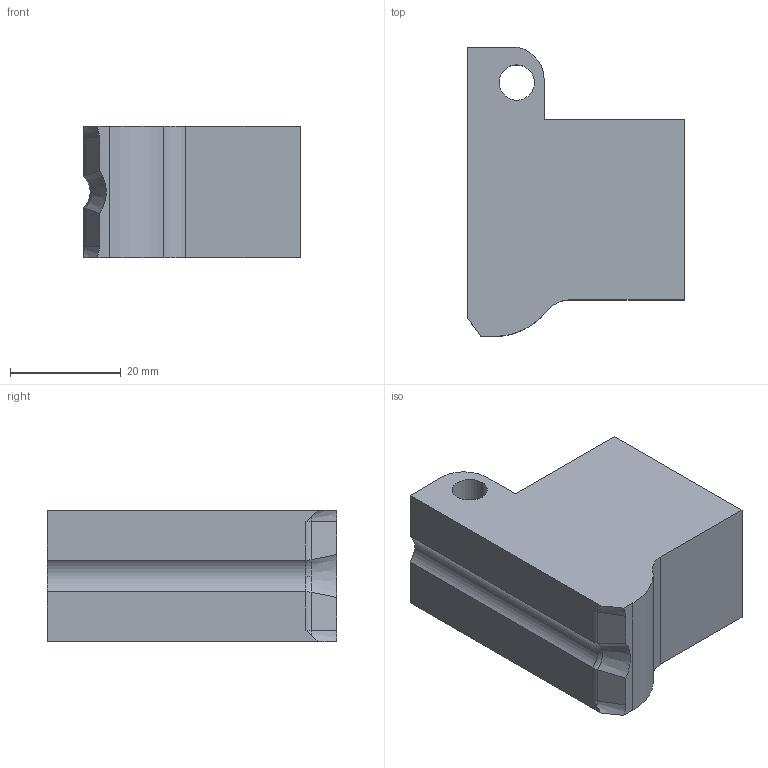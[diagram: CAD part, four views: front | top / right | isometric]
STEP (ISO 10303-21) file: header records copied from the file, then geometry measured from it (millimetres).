
FILE_DESCRIPTION (( 'STEP AP214' ), '1' );
FILE_NAME ('Receiver_Magwell_Front.step', '2014-05-14T06:10:05', ( 'WarFairy' ), ( '' ), 'SwSTEP 2.0', 'SolidWorks 2013', '' );
FILE_SCHEMA (( 'AUTOMOTIVE_DESIGN' ));
Length unit declared in the file: inch
Products named in the file (1): Receiver_Magwell_Front
Bounding box: 39.14 x 52.18 x 23.7 mm (x, y, z)
Volume: 33708 mm3; surface area: 7592.7 mm2
Topology: 1 solids, 1 shells, 34 faces, 90 edges, 58 vertices
Faces by surface type: plane 16, cylinder 11, torus 4, cone 3
Entity records: 1129 total; most frequent: CARTESIAN_POINT 229, ORIENTED_EDGE 180, DIRECTION 179, EDGE_CURVE 90, AXIS2_PLACEMENT_3D 64, VERTEX_POINT 58, VECTOR 51, LINE 51
